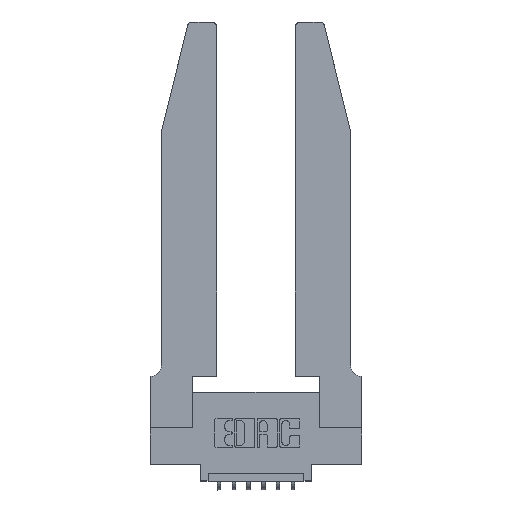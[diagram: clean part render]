
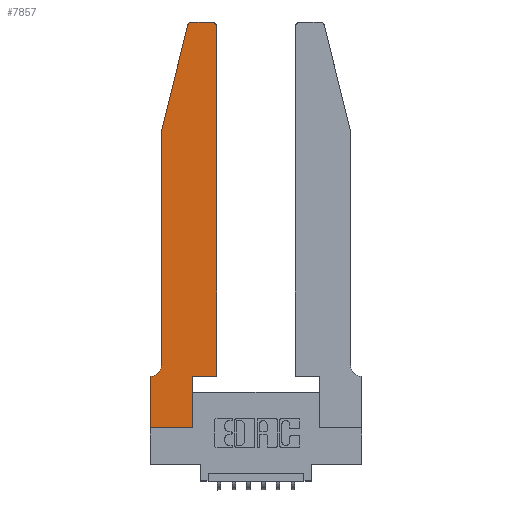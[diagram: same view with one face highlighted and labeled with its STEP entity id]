
A CAD part, top view. The second image highlights one B-rep face of the part: STEP entity #7857.
In plain terms, the highlighted planar face has unit normal (0, 0, 1).
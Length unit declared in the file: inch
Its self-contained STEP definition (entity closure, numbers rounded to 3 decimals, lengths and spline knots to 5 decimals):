
#20 = DIRECTION ( 'NONE',  ( 1., 0., 0. ) ) ;
#53 = CARTESIAN_POINT ( 'NONE',  ( 0.0755, 2., 0.37 ) ) ;
#189 = CARTESIAN_POINT ( 'NONE',  ( 0.0055, 0.42, 0.37 ) ) ;
#224 = VERTEX_POINT ( 'NONE', #653 ) ;
#572 = CARTESIAN_POINT ( 'NONE',  ( 0.2865, 0.35, 0.37 ) ) ;
#580 = DIRECTION ( 'NONE',  ( -1., 0., 0. ) ) ;
#645 = CARTESIAN_POINT ( 'NONE',  ( 0.4505, 2.72, 0.37 ) ) ;
#653 = CARTESIAN_POINT ( 'NONE',  ( 0.0755, 0.42, 0.37 ) ) ;
#663 = AXIS2_PLACEMENT_3D ( 'NONE', #189, #7981, #4687 ) ;
#697 = LINE ( 'NONE', #1731, #3491 ) ;
#803 = CARTESIAN_POINT ( 'NONE',  ( 0., 0., 0.37 ) ) ;
#895 = DIRECTION ( 'NONE',  ( 0., 1., 0. ) ) ;
#1001 = DIRECTION ( 'NONE',  ( 1., 0., 0. ) ) ;
#1229 = VERTEX_POINT ( 'NONE', #8857 ) ;
#1244 = DIRECTION ( 'NONE',  ( 0., 1., 0. ) ) ;
#1346 = ORIENTED_EDGE ( 'NONE', *, *, #9373, .T. ) ;
#1386 = ORIENTED_EDGE ( 'NONE', *, *, #13515, .T. ) ;
#1477 = VERTEX_POINT ( 'NONE', #11113 ) ;
#1515 = ORIENTED_EDGE ( 'NONE', *, *, #13536, .T. ) ;
#1731 = CARTESIAN_POINT ( 'NONE',  ( 0.4505, 0.35, 0.37 ) ) ;
#1864 = LINE ( 'NONE', #10122, #8291 ) ;
#1909 = VERTEX_POINT ( 'NONE', #53 ) ;
#1929 = VERTEX_POINT ( 'NONE', #5603 ) ;
#1984 = CIRCLE ( 'NONE', #4389, 0.03 ) ;
#2030 = VECTOR ( 'NONE', #1001, 39.37008 ) ;
#2089 = LINE ( 'NONE', #8616, #11448 ) ;
#2456 = EDGE_CURVE ( 'NONE', #11786, #8107, #1984, .T. ) ;
#3260 = ORIENTED_EDGE ( 'NONE', *, *, #12023, .T. ) ;
#3333 = DIRECTION ( 'NONE',  ( -1., 0., 0. ) ) ;
#3468 = EDGE_CURVE ( 'NONE', #1477, #13958, #10118, .T. ) ;
#3491 = VECTOR ( 'NONE', #11701, 39.37008 ) ;
#3725 = CARTESIAN_POINT ( 'NONE',  ( 0.25487, 2.72718, 0.37 ) ) ;
#4062 = ORIENTED_EDGE ( 'NONE', *, *, #8798, .T. ) ;
#4158 = DIRECTION ( 'NONE',  ( -0.239, -0.971, 0. ) ) ;
#4389 = AXIS2_PLACEMENT_3D ( 'NONE', #6781, #7908, #20 ) ;
#4424 = CARTESIAN_POINT ( 'NONE',  ( 0.0755, 0.35, 0.37 ) ) ;
#4556 = DIRECTION ( 'NONE',  ( 0., -1., 0. ) ) ;
#4558 = CIRCLE ( 'NONE', #13928, 0.03 ) ;
#4565 = EDGE_CURVE ( 'NONE', #5530, #1909, #2089, .T. ) ;
#4687 = DIRECTION ( 'NONE',  ( -1., 0., 0. ) ) ;
#4870 = VERTEX_POINT ( 'NONE', #572 ) ;
#4907 = ORIENTED_EDGE ( 'NONE', *, *, #12641, .T. ) ;
#5114 = AXIS2_PLACEMENT_3D ( 'NONE', #8932, #13552, #5652 ) ;
#5530 = VERTEX_POINT ( 'NONE', #3725 ) ;
#5603 = CARTESIAN_POINT ( 'NONE',  ( 0.2865, 0., 0.37 ) ) ;
#5652 = DIRECTION ( 'NONE',  ( 1., 0., 0. ) ) ;
#5984 = CARTESIAN_POINT ( 'NONE',  ( 0.2605, 2.75, 0.37 ) ) ;
#6136 = VECTOR ( 'NONE', #4556, 39.37008 ) ;
#6269 = EDGE_CURVE ( 'NONE', #8107, #12977, #8500, .T. ) ;
#6294 = VECTOR ( 'NONE', #3333, 39.37008 ) ;
#6297 = CARTESIAN_POINT ( 'NONE',  ( 0.284, 2.75, 0.37 ) ) ;
#6768 = VECTOR ( 'NONE', #580, 39.37008 ) ;
#6781 = CARTESIAN_POINT ( 'NONE',  ( 0.4205, 2.72, 0.37 ) ) ;
#7501 = LINE ( 'NONE', #14146, #8705 ) ;
#7568 = CARTESIAN_POINT ( 'NONE',  ( 0.4505, 0.35, 0.37 ) ) ;
#7653 = DIRECTION ( 'NONE',  ( 1., 0., 0. ) ) ;
#7796 = LINE ( 'NONE', #13412, #13622 ) ;
#7857 = ADVANCED_FACE ( 'NONE', ( #13325 ), #12115, .T. ) ;
#7901 = LINE ( 'NONE', #12143, #6136 ) ;
#7908 = DIRECTION ( 'NONE',  ( 0., 0., 1. ) ) ;
#7981 = DIRECTION ( 'NONE',  ( 0., 0., -1. ) ) ;
#8058 = ORIENTED_EDGE ( 'NONE', *, *, #9601, .T. ) ;
#8107 = VERTEX_POINT ( 'NONE', #13228 ) ;
#8291 = VECTOR ( 'NONE', #1244, 39.37008 ) ;
#8500 = LINE ( 'NONE', #5984, #6768 ) ;
#8616 = CARTESIAN_POINT ( 'NONE',  ( 0.0755, 2., 0.37 ) ) ;
#8705 = VECTOR ( 'NONE', #895, 39.37008 ) ;
#8798 = EDGE_CURVE ( 'NONE', #13958, #1229, #7796, .T. ) ;
#8857 = CARTESIAN_POINT ( 'NONE',  ( 0., 0., 0.37 ) ) ;
#8932 = CARTESIAN_POINT ( 'NONE',  ( 0., 0.35, 0.37 ) ) ;
#8939 = DIRECTION ( 'NONE',  ( 0., -1., 0. ) ) ;
#9201 = VERTEX_POINT ( 'NONE', #7568 ) ;
#9373 = EDGE_CURVE ( 'NONE', #1229, #1929, #10190, .T. ) ;
#9601 = EDGE_CURVE ( 'NONE', #1929, #4870, #1864, .T. ) ;
#9821 = CARTESIAN_POINT ( 'NONE',  ( 0.284, 2.72, 0.37 ) ) ;
#10118 = LINE ( 'NONE', #4424, #6294 ) ;
#10122 = CARTESIAN_POINT ( 'NONE',  ( 0.2865, 0.35, 0.37 ) ) ;
#10190 = LINE ( 'NONE', #803, #2030 ) ;
#10268 = CIRCLE ( 'NONE', #663, 0.07 ) ;
#10919 = DIRECTION ( 'NONE',  ( 0., 0., 1. ) ) ;
#11113 = CARTESIAN_POINT ( 'NONE',  ( 0.0055, 0.35, 0.37 ) ) ;
#11118 = ORIENTED_EDGE ( 'NONE', *, *, #2456, .T. ) ;
#11448 = VECTOR ( 'NONE', #4158, 39.37008 ) ;
#11502 = ORIENTED_EDGE ( 'NONE', *, *, #13419, .T. ) ;
#11701 = DIRECTION ( 'NONE',  ( 1., 0., 0. ) ) ;
#11786 = VERTEX_POINT ( 'NONE', #645 ) ;
#12023 = EDGE_CURVE ( 'NONE', #1909, #224, #7901, .T. ) ;
#12115 = PLANE ( 'NONE',  #5114 ) ;
#12143 = CARTESIAN_POINT ( 'NONE',  ( 0.0755, 2., 0.37 ) ) ;
#12250 = CARTESIAN_POINT ( 'NONE',  ( 0., 0.35, 0.37 ) ) ;
#12566 = EDGE_LOOP ( 'NONE', ( #13247, #1515, #13685, #3260, #4907, #13682, #4062, #1346, #8058, #11502, #1386, #11118 ) ) ;
#12641 = EDGE_CURVE ( 'NONE', #224, #1477, #10268, .T. ) ;
#12977 = VERTEX_POINT ( 'NONE', #6297 ) ;
#13228 = CARTESIAN_POINT ( 'NONE',  ( 0.4205, 2.75, 0.37 ) ) ;
#13247 = ORIENTED_EDGE ( 'NONE', *, *, #6269, .T. ) ;
#13325 = FACE_OUTER_BOUND ( 'NONE', #12566, .T. ) ;
#13412 = CARTESIAN_POINT ( 'NONE',  ( 0., 0., 0.37 ) ) ;
#13419 = EDGE_CURVE ( 'NONE', #4870, #9201, #697, .T. ) ;
#13515 = EDGE_CURVE ( 'NONE', #9201, #11786, #7501, .T. ) ;
#13536 = EDGE_CURVE ( 'NONE', #12977, #5530, #4558, .T. ) ;
#13552 = DIRECTION ( 'NONE',  ( 0., 0., 1. ) ) ;
#13622 = VECTOR ( 'NONE', #8939, 39.37008 ) ;
#13682 = ORIENTED_EDGE ( 'NONE', *, *, #3468, .T. ) ;
#13685 = ORIENTED_EDGE ( 'NONE', *, *, #4565, .T. ) ;
#13928 = AXIS2_PLACEMENT_3D ( 'NONE', #9821, #10919, #7653 ) ;
#13958 = VERTEX_POINT ( 'NONE', #12250 ) ;
#14146 = CARTESIAN_POINT ( 'NONE',  ( 0.4505, 0.35, 0.37 ) ) ;
